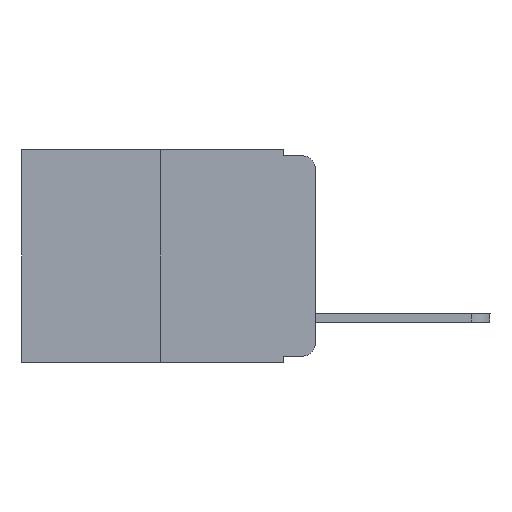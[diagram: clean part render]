
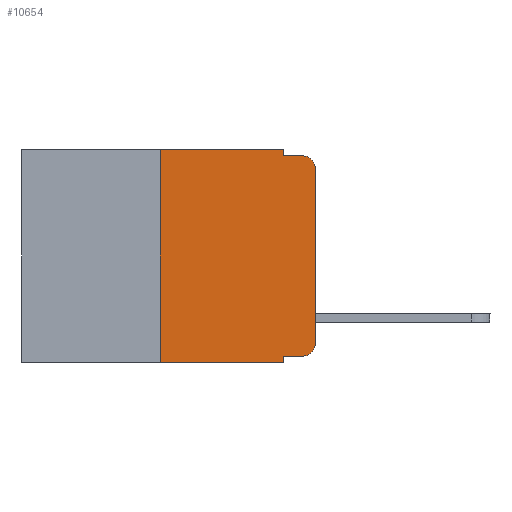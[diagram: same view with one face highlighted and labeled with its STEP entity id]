
A CAD part, left-side view. The second image highlights one B-rep face of the part: STEP entity #10654.
In plain terms, the highlighted planar face has unit normal (-1, 0, 0).
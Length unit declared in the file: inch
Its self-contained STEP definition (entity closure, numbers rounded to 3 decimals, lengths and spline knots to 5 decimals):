
#2 = EDGE_CURVE ( 'NONE', #4870, #3473, #5806, .T. ) ;
#142 = ORIENTED_EDGE ( 'NONE', *, *, #1827, .F. ) ;
#658 = DIRECTION ( 'NONE',  ( 0., -1., 0. ) ) ;
#714 = CARTESIAN_POINT ( 'NONE',  ( 0., 0.051, -0.333 ) ) ;
#769 = LINE ( 'NONE', #3702, #1308 ) ;
#854 = LINE ( 'NONE', #4987, #9549 ) ;
#991 = CARTESIAN_POINT ( 'NONE',  ( 0., 0.02, -0.03 ) ) ;
#1045 = AXIS2_PLACEMENT_3D ( 'NONE', #8567, #3594, #2694 ) ;
#1077 = CARTESIAN_POINT ( 'NONE',  ( 0., 0., 0. ) ) ;
#1086 = VERTEX_POINT ( 'NONE', #2548 ) ;
#1136 = DIRECTION ( 'NONE',  ( -1., 0., 0. ) ) ;
#1308 = VECTOR ( 'NONE', #8676, 39.37008 ) ;
#1827 = EDGE_CURVE ( 'NONE', #6560, #4652, #5521, .T. ) ;
#1860 = ORIENTED_EDGE ( 'NONE', *, *, #8166, .F. ) ;
#1959 = DIRECTION ( 'NONE',  ( 0., -1., 0. ) ) ;
#2020 = VECTOR ( 'NONE', #10164, 39.37008 ) ;
#2133 = AXIS2_PLACEMENT_3D ( 'NONE', #991, #1136, #9291 ) ;
#2262 = EDGE_CURVE ( 'NONE', #10426, #6721, #10128, .T. ) ;
#2517 = ORIENTED_EDGE ( 'NONE', *, *, #9680, .T. ) ;
#2548 = CARTESIAN_POINT ( 'NONE',  ( 0., 0., -0.313 ) ) ;
#2694 = DIRECTION ( 'NONE',  ( 0., 0., -1. ) ) ;
#2717 = ORIENTED_EDGE ( 'NONE', *, *, #4942, .F. ) ;
#2876 = CARTESIAN_POINT ( 'NONE',  ( 0., 0.02, -0.333 ) ) ;
#3056 = CARTESIAN_POINT ( 'NONE',  ( 0., 0.051, 0. ) ) ;
#3062 = LINE ( 'NONE', #3550, #2020 ) ;
#3221 = DIRECTION ( 'NONE',  ( 1., 0., 0. ) ) ;
#3473 = VERTEX_POINT ( 'NONE', #5535 ) ;
#3550 = CARTESIAN_POINT ( 'NONE',  ( 0., 0.051, 0. ) ) ;
#3556 = AXIS2_PLACEMENT_3D ( 'NONE', #7381, #3221, #9849 ) ;
#3594 = DIRECTION ( 'NONE',  ( -1., 0., 0. ) ) ;
#3702 = CARTESIAN_POINT ( 'NONE',  ( 0., 0.051, -0.01 ) ) ;
#4077 = DIRECTION ( 'NONE',  ( 0., -1., 0. ) ) ;
#4122 = CIRCLE ( 'NONE', #1045, 0.02 ) ;
#4336 = ORIENTED_EDGE ( 'NONE', *, *, #2, .T. ) ;
#4449 = VECTOR ( 'NONE', #1959, 39.37008 ) ;
#4652 = VERTEX_POINT ( 'NONE', #9279 ) ;
#4867 = PLANE ( 'NONE',  #3556 ) ;
#4870 = VERTEX_POINT ( 'NONE', #6121 ) ;
#4942 = EDGE_CURVE ( 'NONE', #4652, #3473, #769, .T. ) ;
#4987 = CARTESIAN_POINT ( 'NONE',  ( 0., 0.473, 0. ) ) ;
#5314 = VECTOR ( 'NONE', #6901, 39.37008 ) ;
#5521 = LINE ( 'NONE', #9739, #7203 ) ;
#5535 = CARTESIAN_POINT ( 'NONE',  ( 0., 0.02, -0.01 ) ) ;
#5569 = VECTOR ( 'NONE', #658, 39.37008 ) ;
#5806 = CIRCLE ( 'NONE', #2133, 0.02 ) ;
#6121 = CARTESIAN_POINT ( 'NONE',  ( 0., 0., -0.03 ) ) ;
#6244 = VECTOR ( 'NONE', #7422, 39.37008 ) ;
#6273 = CARTESIAN_POINT ( 'NONE',  ( 0., 0.25, -0.343 ) ) ;
#6560 = VERTEX_POINT ( 'NONE', #3056 ) ;
#6601 = LINE ( 'NONE', #8005, #5569 ) ;
#6721 = VERTEX_POINT ( 'NONE', #7393 ) ;
#6843 = VERTEX_POINT ( 'NONE', #9207 ) ;
#6901 = DIRECTION ( 'NONE',  ( 0., 0., 1. ) ) ;
#6964 = CARTESIAN_POINT ( 'NONE',  ( 0., 0.473, -0.343 ) ) ;
#7203 = VECTOR ( 'NONE', #7261, 39.37008 ) ;
#7261 = DIRECTION ( 'NONE',  ( 0., 0., -1. ) ) ;
#7297 = EDGE_CURVE ( 'NONE', #8810, #9790, #6601, .T. ) ;
#7381 = CARTESIAN_POINT ( 'NONE',  ( 0., 0.473, 0. ) ) ;
#7393 = CARTESIAN_POINT ( 'NONE',  ( 0., 0.051, -0.343 ) ) ;
#7422 = DIRECTION ( 'NONE',  ( 0., 0., 1. ) ) ;
#7454 = CARTESIAN_POINT ( 'NONE',  ( 0., 0.25, 0. ) ) ;
#8005 = CARTESIAN_POINT ( 'NONE',  ( 0., 0.051, -0.333 ) ) ;
#8056 = LINE ( 'NONE', #7454, #6244 ) ;
#8166 = EDGE_CURVE ( 'NONE', #10426, #6843, #8056, .T. ) ;
#8486 = ORIENTED_EDGE ( 'NONE', *, *, #10112, .F. ) ;
#8567 = CARTESIAN_POINT ( 'NONE',  ( 0., 0.02, -0.313 ) ) ;
#8649 = ORIENTED_EDGE ( 'NONE', *, *, #9120, .T. ) ;
#8676 = DIRECTION ( 'NONE',  ( 0., -1., 0. ) ) ;
#8810 = VERTEX_POINT ( 'NONE', #714 ) ;
#9120 = EDGE_CURVE ( 'NONE', #1086, #4870, #9710, .T. ) ;
#9207 = CARTESIAN_POINT ( 'NONE',  ( 0., 0.25, 0. ) ) ;
#9279 = CARTESIAN_POINT ( 'NONE',  ( 0., 0.051, -0.01 ) ) ;
#9291 = DIRECTION ( 'NONE',  ( 0., 0., -1. ) ) ;
#9549 = VECTOR ( 'NONE', #4077, 39.37008 ) ;
#9680 = EDGE_CURVE ( 'NONE', #9790, #1086, #4122, .T. ) ;
#9710 = LINE ( 'NONE', #1077, #5314 ) ;
#9739 = CARTESIAN_POINT ( 'NONE',  ( 0., 0.051, 0. ) ) ;
#9766 = ORIENTED_EDGE ( 'NONE', *, *, #10327, .F. ) ;
#9790 = VERTEX_POINT ( 'NONE', #2876 ) ;
#9849 = DIRECTION ( 'NONE',  ( 0., 0., -1. ) ) ;
#10032 = ORIENTED_EDGE ( 'NONE', *, *, #7297, .T. ) ;
#10112 = EDGE_CURVE ( 'NONE', #6843, #6560, #854, .T. ) ;
#10128 = LINE ( 'NONE', #6964, #4449 ) ;
#10162 = FACE_OUTER_BOUND ( 'NONE', #10234, .T. ) ;
#10164 = DIRECTION ( 'NONE',  ( 0., 0., -1. ) ) ;
#10234 = EDGE_LOOP ( 'NONE', ( #8649, #4336, #2717, #142, #8486, #1860, #10644, #9766, #10032, #2517 ) ) ;
#10327 = EDGE_CURVE ( 'NONE', #8810, #6721, #3062, .T. ) ;
#10426 = VERTEX_POINT ( 'NONE', #6273 ) ;
#10644 = ORIENTED_EDGE ( 'NONE', *, *, #2262, .T. ) ;
#10654 = ADVANCED_FACE ( 'NONE', ( #10162 ), #4867, .F. ) ;
